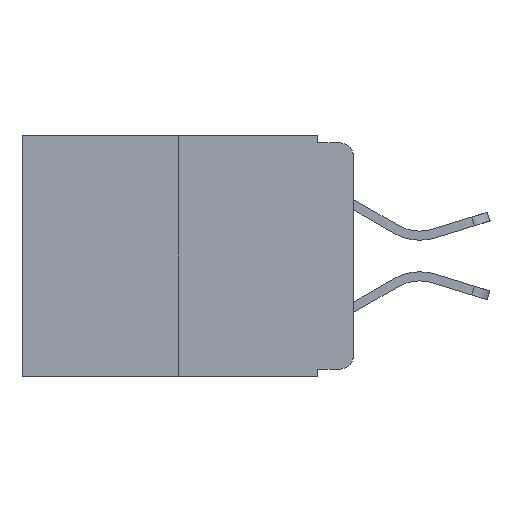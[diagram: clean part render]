
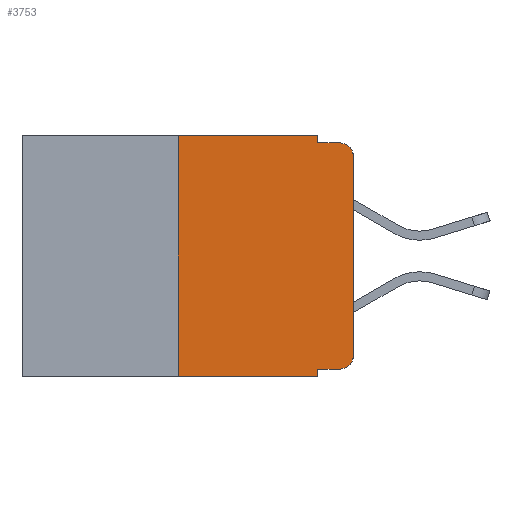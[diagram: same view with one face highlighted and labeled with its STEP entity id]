
A CAD part, left-side view. The second image highlights one B-rep face of the part: STEP entity #3753.
In plain terms, the highlighted planar face has unit normal (-1, 0, 0).
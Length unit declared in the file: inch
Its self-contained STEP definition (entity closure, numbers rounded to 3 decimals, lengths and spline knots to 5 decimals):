
#158 = VECTOR ( 'NONE', #18526, 39.37008 ) ;
#509 = DIRECTION ( 'NONE',  ( -1., 0., 0. ) ) ;
#788 = DIRECTION ( 'NONE',  ( 0., 0., 1. ) ) ;
#1051 = LINE ( 'NONE', #7103, #5327 ) ;
#1151 = VERTEX_POINT ( 'NONE', #24645 ) ;
#1245 = DIRECTION ( 'NONE',  ( 0., 0., 1. ) ) ;
#1399 = VECTOR ( 'NONE', #22422, 39.37008 ) ;
#1918 = CARTESIAN_POINT ( 'NONE',  ( 0., 0.051, 0. ) ) ;
#2189 = VERTEX_POINT ( 'NONE', #25458 ) ;
#2233 = ORIENTED_EDGE ( 'NONE', *, *, #13468, .T. ) ;
#2354 = EDGE_CURVE ( 'NONE', #1151, #4285, #3405, .T. ) ;
#2511 = DIRECTION ( 'NONE',  ( -1., 0., 0. ) ) ;
#3309 = CARTESIAN_POINT ( 'NONE',  ( 0., 0.051, 0. ) ) ;
#3405 = LINE ( 'NONE', #3309, #24693 ) ;
#3703 = LINE ( 'NONE', #21402, #19570 ) ;
#3753 = ADVANCED_FACE ( 'NONE', ( #11112 ), #16382, .F. ) ;
#3933 = CARTESIAN_POINT ( 'NONE',  ( 0., 0.051, -0.01 ) ) ;
#4285 = VERTEX_POINT ( 'NONE', #3933 ) ;
#5090 = CARTESIAN_POINT ( 'NONE',  ( 0., 0.051, -0.343 ) ) ;
#5327 = VECTOR ( 'NONE', #788, 39.37008 ) ;
#5462 = CARTESIAN_POINT ( 'NONE',  ( 0., 0.051, -0.01 ) ) ;
#5740 = LINE ( 'NONE', #1918, #158 ) ;
#5814 = ORIENTED_EDGE ( 'NONE', *, *, #9305, .F. ) ;
#5900 = LINE ( 'NONE', #19738, #26463 ) ;
#6044 = DIRECTION ( 'NONE',  ( 1., 0., 0. ) ) ;
#6090 = AXIS2_PLACEMENT_3D ( 'NONE', #18437, #6044, #20491 ) ;
#7103 = CARTESIAN_POINT ( 'NONE',  ( 0., 0.25, 0. ) ) ;
#7550 = DIRECTION ( 'NONE',  ( 0., -1., 0. ) ) ;
#7570 = EDGE_CURVE ( 'NONE', #20268, #1151, #15845, .T. ) ;
#7602 = CARTESIAN_POINT ( 'NONE',  ( 0., 0.051, -0.333 ) ) ;
#8238 = EDGE_LOOP ( 'NONE', ( #17143, #2233, #5814, #13411, #11498, #16040, #8327, #22707, #9365, #25183 ) ) ;
#8318 = CIRCLE ( 'NONE', #19498, 0.02 ) ;
#8327 = ORIENTED_EDGE ( 'NONE', *, *, #20957, .T. ) ;
#8340 = VERTEX_POINT ( 'NONE', #16835 ) ;
#9051 = DIRECTION ( 'NONE',  ( 0., -1., 0. ) ) ;
#9081 = VERTEX_POINT ( 'NONE', #15067 ) ;
#9305 = EDGE_CURVE ( 'NONE', #4285, #19415, #9625, .T. ) ;
#9365 = ORIENTED_EDGE ( 'NONE', *, *, #11214, .T. ) ;
#9625 = LINE ( 'NONE', #5462, #24753 ) ;
#9817 = EDGE_CURVE ( 'NONE', #9081, #15276, #8318, .T. ) ;
#11112 = FACE_OUTER_BOUND ( 'NONE', #8238, .T. ) ;
#11214 = EDGE_CURVE ( 'NONE', #24548, #9081, #22120, .T. ) ;
#11498 = ORIENTED_EDGE ( 'NONE', *, *, #7570, .F. ) ;
#11594 = VERTEX_POINT ( 'NONE', #5090 ) ;
#11674 = CIRCLE ( 'NONE', #16104, 0.02 ) ;
#12206 = DIRECTION ( 'NONE',  ( 0., -1., 0. ) ) ;
#12972 = CARTESIAN_POINT ( 'NONE',  ( 0., 0.02, -0.03 ) ) ;
#13411 = ORIENTED_EDGE ( 'NONE', *, *, #2354, .F. ) ;
#13468 = EDGE_CURVE ( 'NONE', #2189, #19415, #11674, .T. ) ;
#14589 = CARTESIAN_POINT ( 'NONE',  ( 0., 0.25, 0. ) ) ;
#14932 = CARTESIAN_POINT ( 'NONE',  ( 0., 0.02, -0.313 ) ) ;
#15067 = CARTESIAN_POINT ( 'NONE',  ( 0., 0.02, -0.333 ) ) ;
#15069 = DIRECTION ( 'NONE',  ( 0., 0., -1. ) ) ;
#15276 = VERTEX_POINT ( 'NONE', #16848 ) ;
#15845 = LINE ( 'NONE', #18469, #21311 ) ;
#16040 = ORIENTED_EDGE ( 'NONE', *, *, #22245, .F. ) ;
#16104 = AXIS2_PLACEMENT_3D ( 'NONE', #12972, #509, #15069 ) ;
#16258 = EDGE_CURVE ( 'NONE', #15276, #2189, #5900, .T. ) ;
#16382 = PLANE ( 'NONE',  #6090 ) ;
#16835 = CARTESIAN_POINT ( 'NONE',  ( 0., 0.25, -0.343 ) ) ;
#16848 = CARTESIAN_POINT ( 'NONE',  ( 0., 0., -0.313 ) ) ;
#17043 = DIRECTION ( 'NONE',  ( 0., 0., -1. ) ) ;
#17143 = ORIENTED_EDGE ( 'NONE', *, *, #16258, .T. ) ;
#17806 = DIRECTION ( 'NONE',  ( 0., 0., -1. ) ) ;
#18162 = CARTESIAN_POINT ( 'NONE',  ( 0., 0.02, -0.01 ) ) ;
#18437 = CARTESIAN_POINT ( 'NONE',  ( 0., 0.473, 0. ) ) ;
#18469 = CARTESIAN_POINT ( 'NONE',  ( 0., 0.473, 0. ) ) ;
#18526 = DIRECTION ( 'NONE',  ( 0., 0., -1. ) ) ;
#19415 = VERTEX_POINT ( 'NONE', #18162 ) ;
#19498 = AXIS2_PLACEMENT_3D ( 'NONE', #14932, #2511, #17043 ) ;
#19525 = EDGE_CURVE ( 'NONE', #24548, #11594, #5740, .T. ) ;
#19570 = VECTOR ( 'NONE', #9051, 39.37008 ) ;
#19738 = CARTESIAN_POINT ( 'NONE',  ( 0., 0., 0. ) ) ;
#20268 = VERTEX_POINT ( 'NONE', #14589 ) ;
#20491 = DIRECTION ( 'NONE',  ( 0., 0., -1. ) ) ;
#20957 = EDGE_CURVE ( 'NONE', #8340, #11594, #3703, .T. ) ;
#21311 = VECTOR ( 'NONE', #12206, 39.37008 ) ;
#21402 = CARTESIAN_POINT ( 'NONE',  ( 0., 0.473, -0.343 ) ) ;
#22120 = LINE ( 'NONE', #26385, #1399 ) ;
#22245 = EDGE_CURVE ( 'NONE', #8340, #20268, #1051, .T. ) ;
#22422 = DIRECTION ( 'NONE',  ( 0., -1., 0. ) ) ;
#22707 = ORIENTED_EDGE ( 'NONE', *, *, #19525, .F. ) ;
#24548 = VERTEX_POINT ( 'NONE', #7602 ) ;
#24645 = CARTESIAN_POINT ( 'NONE',  ( 0., 0.051, 0. ) ) ;
#24693 = VECTOR ( 'NONE', #17806, 39.37008 ) ;
#24753 = VECTOR ( 'NONE', #7550, 39.37008 ) ;
#25183 = ORIENTED_EDGE ( 'NONE', *, *, #9817, .T. ) ;
#25458 = CARTESIAN_POINT ( 'NONE',  ( 0., 0., -0.03 ) ) ;
#26385 = CARTESIAN_POINT ( 'NONE',  ( 0., 0.051, -0.333 ) ) ;
#26463 = VECTOR ( 'NONE', #1245, 39.37008 ) ;
